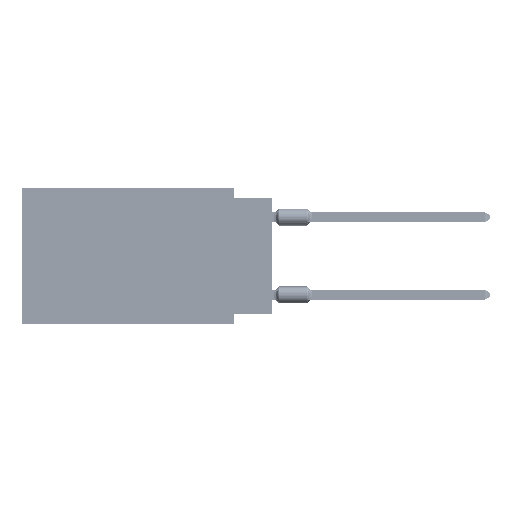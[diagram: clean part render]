
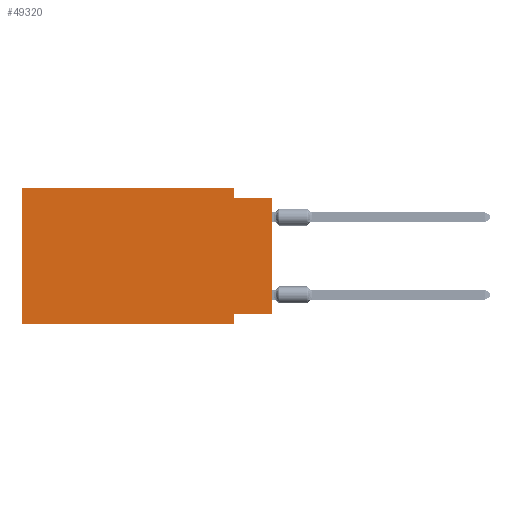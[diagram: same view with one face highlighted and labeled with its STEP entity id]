
A CAD part, left-side view. The second image highlights one B-rep face of the part: STEP entity #49320.
In plain terms, the highlighted planar face has unit normal (-1, 0, 0).
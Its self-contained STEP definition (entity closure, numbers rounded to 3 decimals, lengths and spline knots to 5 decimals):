
#527 = VERTEX_POINT ( 'NONE', #31063 ) ;
#1607 = VECTOR ( 'NONE', #19446, 39.37008 ) ;
#2923 = DIRECTION ( 'NONE',  ( 0., -1., 0. ) ) ;
#4838 = CARTESIAN_POINT ( 'NONE',  ( 0., 0.1, 0. ) ) ;
#5692 = ORIENTED_EDGE ( 'NONE', *, *, #36256, .F. ) ;
#9197 = VECTOR ( 'NONE', #73672, 39.37008 ) ;
#10412 = CARTESIAN_POINT ( 'NONE',  ( 0., 0.645, 0. ) ) ;
#12387 = VECTOR ( 'NONE', #38898, 39.37008 ) ;
#13616 = CARTESIAN_POINT ( 'NONE',  ( 0., 0., -0.325 ) ) ;
#14779 = LINE ( 'NONE', #37945, #12387 ) ;
#15214 = LINE ( 'NONE', #30173, #9197 ) ;
#19425 = EDGE_CURVE ( 'NONE', #527, #37052, #55649, .T. ) ;
#19446 = DIRECTION ( 'NONE',  ( 0., 1., 0. ) ) ;
#20486 = VECTOR ( 'NONE', #87918, 39.37008 ) ;
#20880 = VERTEX_POINT ( 'NONE', #22938 ) ;
#20906 = VERTEX_POINT ( 'NONE', #59672 ) ;
#22744 = DIRECTION ( 'NONE',  ( 1., 0., 0. ) ) ;
#22938 = CARTESIAN_POINT ( 'NONE',  ( 0., 0.645, 0. ) ) ;
#23219 = DIRECTION ( 'NONE',  ( 0., 0., -1. ) ) ;
#23241 = VECTOR ( 'NONE', #39884, 39.37008 ) ;
#23248 = VERTEX_POINT ( 'NONE', #4838 ) ;
#23976 = EDGE_CURVE ( 'NONE', #527, #20880, #47125, .T. ) ;
#24444 = EDGE_CURVE ( 'NONE', #73663, #20906, #76375, .T. ) ;
#26216 = CARTESIAN_POINT ( 'NONE',  ( 0., 0., -0.325 ) ) ;
#27309 = ORIENTED_EDGE ( 'NONE', *, *, #51390, .T. ) ;
#29966 = ORIENTED_EDGE ( 'NONE', *, *, #24444, .F. ) ;
#30173 = CARTESIAN_POINT ( 'NONE',  ( 0., 0.645, 0. ) ) ;
#31063 = CARTESIAN_POINT ( 'NONE',  ( 0., 0.645, -0.35 ) ) ;
#31524 = CARTESIAN_POINT ( 'NONE',  ( 0., 0.1, -0.35 ) ) ;
#34773 = CARTESIAN_POINT ( 'NONE',  ( 0., 0.1, -0.025 ) ) ;
#35094 = AXIS2_PLACEMENT_3D ( 'NONE', #59483, #22744, #23219 ) ;
#36256 = EDGE_CURVE ( 'NONE', #20880, #23248, #15214, .T. ) ;
#37052 = VERTEX_POINT ( 'NONE', #31524 ) ;
#37283 = EDGE_CURVE ( 'NONE', #49193, #56658, #57584, .T. ) ;
#37945 = CARTESIAN_POINT ( 'NONE',  ( 0., 0.1, 0. ) ) ;
#38898 = DIRECTION ( 'NONE',  ( 0., 0., -1. ) ) ;
#39676 = ORIENTED_EDGE ( 'NONE', *, *, #19425, .T. ) ;
#39884 = DIRECTION ( 'NONE',  ( 0., 0., 1. ) ) ;
#42559 = DIRECTION ( 'NONE',  ( 0., -1., 0. ) ) ;
#44278 = EDGE_CURVE ( 'NONE', #56658, #37052, #80667, .T. ) ;
#47125 = LINE ( 'NONE', #10412, #23241 ) ;
#49193 = VERTEX_POINT ( 'NONE', #26216 ) ;
#49320 = ADVANCED_FACE ( 'NONE', ( #89406 ), #58064, .F. ) ;
#50600 = LINE ( 'NONE', #88264, #67568 ) ;
#51390 = EDGE_CURVE ( 'NONE', #49193, #20906, #50600, .T. ) ;
#52828 = EDGE_CURVE ( 'NONE', #23248, #73663, #14779, .T. ) ;
#53477 = EDGE_LOOP ( 'NONE', ( #27309, #29966, #63618, #5692, #84357, #39676, #57271, #90998 ) ) ;
#55649 = LINE ( 'NONE', #79289, #82763 ) ;
#56658 = VERTEX_POINT ( 'NONE', #66597 ) ;
#57271 = ORIENTED_EDGE ( 'NONE', *, *, #44278, .F. ) ;
#57584 = LINE ( 'NONE', #13616, #1607 ) ;
#58064 = PLANE ( 'NONE',  #35094 ) ;
#59483 = CARTESIAN_POINT ( 'NONE',  ( 0., 0.645, 0. ) ) ;
#59672 = CARTESIAN_POINT ( 'NONE',  ( 0., 0., -0.025 ) ) ;
#63618 = ORIENTED_EDGE ( 'NONE', *, *, #52828, .F. ) ;
#66182 = CARTESIAN_POINT ( 'NONE',  ( 0., 0.1, -0.35 ) ) ;
#66597 = CARTESIAN_POINT ( 'NONE',  ( 0., 0.1, -0.325 ) ) ;
#67568 = VECTOR ( 'NONE', #80548, 39.37008 ) ;
#69128 = CARTESIAN_POINT ( 'NONE',  ( 0., 0., -0.025 ) ) ;
#73663 = VERTEX_POINT ( 'NONE', #34773 ) ;
#73672 = DIRECTION ( 'NONE',  ( 0., -1., 0. ) ) ;
#76375 = LINE ( 'NONE', #69128, #94069 ) ;
#79289 = CARTESIAN_POINT ( 'NONE',  ( 0., 0.645, -0.35 ) ) ;
#80548 = DIRECTION ( 'NONE',  ( 0., 0., 1. ) ) ;
#80667 = LINE ( 'NONE', #66182, #20486 ) ;
#82763 = VECTOR ( 'NONE', #42559, 39.37008 ) ;
#84357 = ORIENTED_EDGE ( 'NONE', *, *, #23976, .F. ) ;
#87918 = DIRECTION ( 'NONE',  ( 0., 0., -1. ) ) ;
#88264 = CARTESIAN_POINT ( 'NONE',  ( 0., 0., 0. ) ) ;
#89406 = FACE_OUTER_BOUND ( 'NONE', #53477, .T. ) ;
#90998 = ORIENTED_EDGE ( 'NONE', *, *, #37283, .F. ) ;
#94069 = VECTOR ( 'NONE', #2923, 39.37008 ) ;
